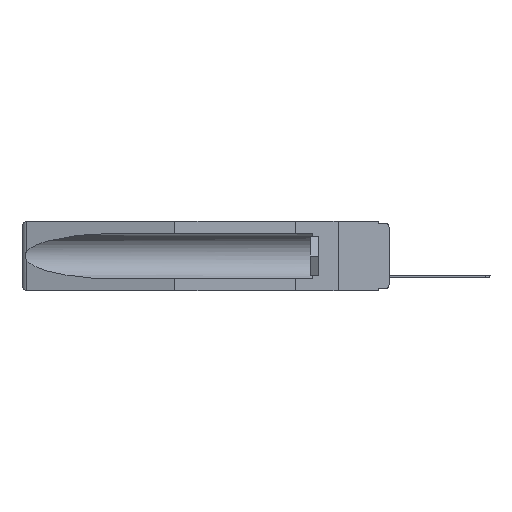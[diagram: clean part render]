
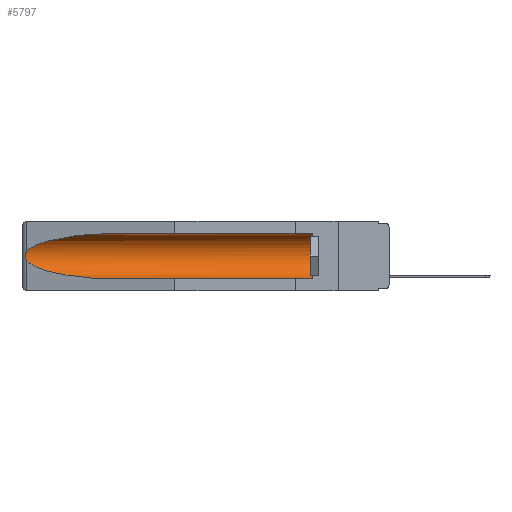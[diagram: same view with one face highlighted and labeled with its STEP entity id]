
A CAD part, left-side view. The second image highlights one B-rep face of the part: STEP entity #5797.
In plain terms, the highlighted cylindrical face has radius 2.857 mm (diameter 5.715 mm), a partial arc.
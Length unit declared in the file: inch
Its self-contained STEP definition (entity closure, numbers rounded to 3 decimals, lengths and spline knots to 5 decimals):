
#43 = AXIS2_PLACEMENT_3D ( 'NONE', #3123, #19229, #1845 ) ;
#384 = DIRECTION ( 'NONE',  ( 0., 1., 0. ) ) ;
#1537 = VECTOR ( 'NONE', #384, 39.37008 ) ;
#1845 = DIRECTION ( 'NONE',  ( 0., 0., 1. ) ) ;
#2410 =( BOUNDED_CURVE ( )  B_SPLINE_CURVE ( 3, ( #17338, #14111, #11218, #12677 ),
 .UNSPECIFIED., .F., .T. ) 
 B_SPLINE_CURVE_WITH_KNOTS ( ( 4, 4 ),
 ( 0.1948, 1.5708 ),
 .UNSPECIFIED. ) 
 CURVE ( )  GEOMETRIC_REPRESENTATION_ITEM ( )  RATIONAL_B_SPLINE_CURVE ( ( 1., 0.848, 0.848, 1. ) ) 
 REPRESENTATION_ITEM ( '' )  );
#2996 = ORIENTED_EDGE ( 'NONE', *, *, #11668, .T. ) ;
#3103 = ORIENTED_EDGE ( 'NONE', *, *, #9381, .T. ) ;
#3123 = CARTESIAN_POINT ( 'NONE',  ( 0.155, -0.30754, -0.1715 ) ) ;
#3231 = FACE_OUTER_BOUND ( 'NONE', #7318, .T. ) ;
#3374 = ORIENTED_EDGE ( 'NONE', *, *, #7133, .T. ) ;
#3445 = CYLINDRICAL_SURFACE ( 'NONE', #43, 0.1125 ) ;
#3804 = DIRECTION ( 'NONE',  ( 0., 0., 1. ) ) ;
#4119 = CARTESIAN_POINT ( 'NONE',  ( 0.26537, 1.52718, -0.19328 ) ) ;
#4840 = CARTESIAN_POINT ( 'NONE',  ( 0.155, 1.07973, -0.059 ) ) ;
#4917 = CARTESIAN_POINT ( 'NONE',  ( 0.21114, 1.30732, -0.059 ) ) ;
#4957 = VERTEX_POINT ( 'NONE', #9948 ) ;
#5797 = ADVANCED_FACE ( 'NONE', ( #3231 ), #3445, .F. ) ;
#5991 = B_SPLINE_CURVE_WITH_KNOTS ( 'NONE', 3,
 ( #15246, #20134, #15149, #20428, #7301, #20330, #10530, #12016, #13847, #17176 ),
 .UNSPECIFIED., .F., .F.,
 ( 4, 2, 2, 2, 4 ),
 ( 0., 0.00029, 0.00058, 0.00087, 0.00117 ),
 .UNSPECIFIED. ) ;
#6285 = VERTEX_POINT ( 'NONE', #14832 ) ;
#6398 = DIRECTION ( 'NONE',  ( 0., 1., 0. ) ) ;
#7055 = DIRECTION ( 'NONE',  ( 0., -1., 0. ) ) ;
#7133 = EDGE_CURVE ( 'NONE', #7761, #6285, #10209, .T. ) ;
#7301 = CARTESIAN_POINT ( 'NONE',  ( 0.2675, 1.53308, -0.16763 ) ) ;
#7318 = EDGE_LOOP ( 'NONE', ( #3374, #3103, #2996, #10709, #15216, #10936 ) ) ;
#7628 = VECTOR ( 'NONE', #6398, 39.37008 ) ;
#7761 = VERTEX_POINT ( 'NONE', #4840 ) ;
#7977 = LINE ( 'NONE', #20829, #7628 ) ;
#8730 = CARTESIAN_POINT ( 'NONE',  ( 0.155, 0.126, -0.1715 ) ) ;
#8928 = EDGE_CURVE ( 'NONE', #13150, #7761, #16781, .T. ) ;
#9381 = EDGE_CURVE ( 'NONE', #6285, #19284, #5991, .T. ) ;
#9948 = CARTESIAN_POINT ( 'NONE',  ( 0.155, 0.126, -0.284 ) ) ;
#10060 = CARTESIAN_POINT ( 'NONE',  ( 0.155, -0.30754, -0.059 ) ) ;
#10209 =( BOUNDED_CURVE ( )  B_SPLINE_CURVE ( 3, ( #14411, #4917, #11310, #12551 ),
 .UNSPECIFIED., .F., .T. ) 
 B_SPLINE_CURVE_WITH_KNOTS ( ( 4, 4 ),
 ( 4.71239, 6.08839 ),
 .UNSPECIFIED. ) 
 CURVE ( )  GEOMETRIC_REPRESENTATION_ITEM ( )  RATIONAL_B_SPLINE_CURVE ( ( 1., 0.848, 0.848, 1. ) ) 
 REPRESENTATION_ITEM ( '' )  );
#10530 = CARTESIAN_POINT ( 'NONE',  ( 0.2673, 1.53269, -0.17917 ) ) ;
#10709 = ORIENTED_EDGE ( 'NONE', *, *, #11733, .F. ) ;
#10936 = ORIENTED_EDGE ( 'NONE', *, *, #8928, .T. ) ;
#11218 = CARTESIAN_POINT ( 'NONE',  ( 0.21114, 1.30732, -0.284 ) ) ;
#11310 = CARTESIAN_POINT ( 'NONE',  ( 0.25451, 1.48313, -0.09465 ) ) ;
#11668 = EDGE_CURVE ( 'NONE', #19284, #17465, #2410, .T. ) ;
#11733 = EDGE_CURVE ( 'NONE', #4957, #17465, #7977, .T. ) ;
#12016 = CARTESIAN_POINT ( 'NONE',  ( 0.26655, 1.53094, -0.18657 ) ) ;
#12551 = CARTESIAN_POINT ( 'NONE',  ( 0.26537, 1.52718, -0.14972 ) ) ;
#12677 = CARTESIAN_POINT ( 'NONE',  ( 0.155, 1.07973, -0.284 ) ) ;
#13150 = VERTEX_POINT ( 'NONE', #19812 ) ;
#13847 = CARTESIAN_POINT ( 'NONE',  ( 0.26597, 1.5296, -0.19026 ) ) ;
#14111 = CARTESIAN_POINT ( 'NONE',  ( 0.25451, 1.48313, -0.24835 ) ) ;
#14411 = CARTESIAN_POINT ( 'NONE',  ( 0.155, 1.07973, -0.059 ) ) ;
#14832 = CARTESIAN_POINT ( 'NONE',  ( 0.26537, 1.52718, -0.14972 ) ) ;
#14853 = EDGE_CURVE ( 'NONE', #4957, #13150, #18891, .T. ) ;
#15149 = CARTESIAN_POINT ( 'NONE',  ( 0.26654, 1.53092, -0.15636 ) ) ;
#15216 = ORIENTED_EDGE ( 'NONE', *, *, #14853, .T. ) ;
#15246 = CARTESIAN_POINT ( 'NONE',  ( 0.26537, 1.52718, -0.14972 ) ) ;
#16336 = CARTESIAN_POINT ( 'NONE',  ( 0.155, 1.07973, -0.284 ) ) ;
#16781 = LINE ( 'NONE', #10060, #1537 ) ;
#17176 = CARTESIAN_POINT ( 'NONE',  ( 0.26537, 1.52718, -0.19328 ) ) ;
#17338 = CARTESIAN_POINT ( 'NONE',  ( 0.26537, 1.52718, -0.19328 ) ) ;
#17465 = VERTEX_POINT ( 'NONE', #16336 ) ;
#18891 = CIRCLE ( 'NONE', #19248, 0.1125 ) ;
#19229 = DIRECTION ( 'NONE',  ( 0., 1., 0. ) ) ;
#19248 = AXIS2_PLACEMENT_3D ( 'NONE', #8730, #7055, #3804 ) ;
#19284 = VERTEX_POINT ( 'NONE', #4119 ) ;
#19812 = CARTESIAN_POINT ( 'NONE',  ( 0.155, 0.126, -0.059 ) ) ;
#20134 = CARTESIAN_POINT ( 'NONE',  ( 0.26597, 1.52961, -0.15275 ) ) ;
#20330 = CARTESIAN_POINT ( 'NONE',  ( 0.2675, 1.53308, -0.17534 ) ) ;
#20428 = CARTESIAN_POINT ( 'NONE',  ( 0.2673, 1.5327, -0.16383 ) ) ;
#20829 = CARTESIAN_POINT ( 'NONE',  ( 0.155, -0.30754, -0.284 ) ) ;
